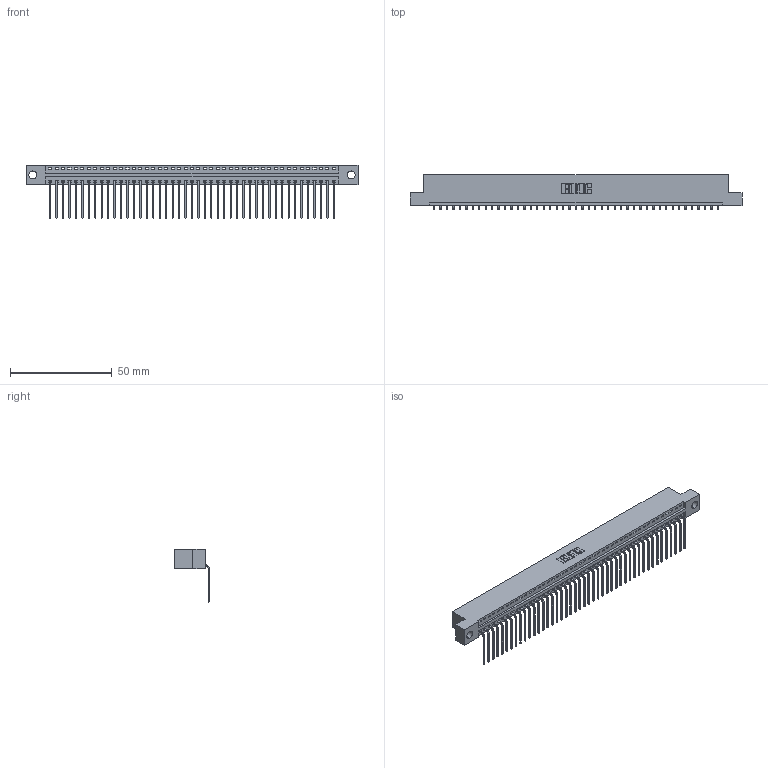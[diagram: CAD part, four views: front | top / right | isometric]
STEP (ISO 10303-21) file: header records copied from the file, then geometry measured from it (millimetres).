
FILE_DESCRIPTION (( 'STEP AP203' ), '1' );
FILE_NAME ('346-045-559-104.STEP', '2022-05-09T19:13:04', ( '' ), ( '' ), 'SwSTEP 2.0', 'SolidWorks 2020', '' );
FILE_SCHEMA (( 'CONFIG_CONTROL_DESIGN' ));
Length unit declared in the file: inch
Products named in the file (3): 346 Part_Flush Mounting Lugs - 0.156 Dia-TH; 346-045-559-104; 345-292-001_558 559 Tail - 1
Assembly tree (46 placements, depth 2):
  346-045-559-104
    346 Part_Flush Mounting Lugs - 0.156 Dia-TH
    345-292-001_558 559 Tail - 1  x45
Bounding box: 163.45 x 17.08 x 26.16 mm (x, y, z)
Volume: 15710.3 mm3; surface area: 20400 mm2
Topology: 46 solids, 46 shells, 2836 faces, 8555 edges, 5642 vertices
Faces by surface type: plane 1980, cylinder 856
Entity records: 28027 total; most frequent: CARTESIAN_POINT 4813, ORIENTED_EDGE 4790, DIRECTION 4241, EDGE_CURVE 2395, VECTOR 2083, LINE 2083, VERTEX_POINT 1594, AXIS2_PLACEMENT_3D 1079
